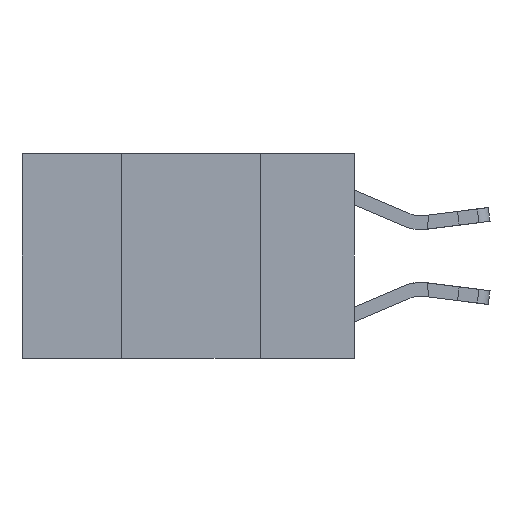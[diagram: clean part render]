
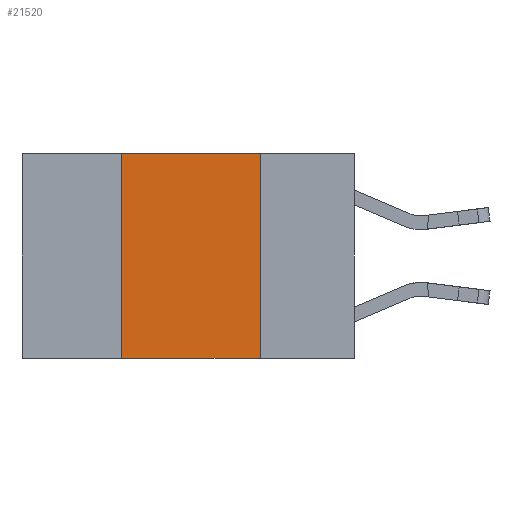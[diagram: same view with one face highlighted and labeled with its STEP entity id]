
A CAD part, left-side view. The second image highlights one B-rep face of the part: STEP entity #21520.
In plain terms, the highlighted planar face has unit normal (-1, 0, 0).
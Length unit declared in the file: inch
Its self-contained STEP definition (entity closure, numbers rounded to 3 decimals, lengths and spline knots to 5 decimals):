
#1584 = DIRECTION ( 'NONE',  ( 0., 0., 1. ) ) ;
#1764 = CARTESIAN_POINT ( 'NONE',  ( 0., 0.6, 0. ) ) ;
#3880 = AXIS2_PLACEMENT_3D ( 'NONE', #1764, #25860, #23406 ) ;
#3926 = PLANE ( 'NONE',  #3880 ) ;
#3977 = VERTEX_POINT ( 'NONE', #17524 ) ;
#4005 = LINE ( 'NONE', #19149, #17135 ) ;
#4527 = VERTEX_POINT ( 'NONE', #25700 ) ;
#5379 = CARTESIAN_POINT ( 'NONE',  ( 0., 0.6, 0. ) ) ;
#5884 = LINE ( 'NONE', #21220, #24998 ) ;
#6256 = ORIENTED_EDGE ( 'NONE', *, *, #8584, .F. ) ;
#6330 = EDGE_LOOP ( 'NONE', ( #6256, #14389, #12923, #17954 ) ) ;
#7121 = DIRECTION ( 'NONE',  ( 0., 0., -1. ) ) ;
#7507 = DIRECTION ( 'NONE',  ( 0., -1., 0. ) ) ;
#8006 = EDGE_CURVE ( 'NONE', #17772, #4527, #5884, .T. ) ;
#8355 = CARTESIAN_POINT ( 'NONE',  ( 0., 0.17, -0.37 ) ) ;
#8414 = EDGE_CURVE ( 'NONE', #17772, #23337, #4005, .T. ) ;
#8584 = EDGE_CURVE ( 'NONE', #3977, #23337, #15847, .T. ) ;
#10633 = FACE_OUTER_BOUND ( 'NONE', #6330, .T. ) ;
#12923 = ORIENTED_EDGE ( 'NONE', *, *, #8006, .F. ) ;
#13916 = CARTESIAN_POINT ( 'NONE',  ( 0., 0.42, -0.37 ) ) ;
#14389 = ORIENTED_EDGE ( 'NONE', *, *, #17195, .F. ) ;
#15847 = LINE ( 'NONE', #17856, #17683 ) ;
#16482 = VECTOR ( 'NONE', #7507, 39.37008 ) ;
#17135 = VECTOR ( 'NONE', #23484, 39.37008 ) ;
#17195 = EDGE_CURVE ( 'NONE', #4527, #3977, #27039, .T. ) ;
#17524 = CARTESIAN_POINT ( 'NONE',  ( 0., 0.17, 0. ) ) ;
#17683 = VECTOR ( 'NONE', #7121, 39.37008 ) ;
#17772 = VERTEX_POINT ( 'NONE', #13916 ) ;
#17856 = CARTESIAN_POINT ( 'NONE',  ( 0., 0.17, 0. ) ) ;
#17954 = ORIENTED_EDGE ( 'NONE', *, *, #8414, .T. ) ;
#19149 = CARTESIAN_POINT ( 'NONE',  ( 0., 0.6, -0.37 ) ) ;
#21220 = CARTESIAN_POINT ( 'NONE',  ( 0., 0.42, 0. ) ) ;
#21520 = ADVANCED_FACE ( 'NONE', ( #10633 ), #3926, .F. ) ;
#23337 = VERTEX_POINT ( 'NONE', #8355 ) ;
#23406 = DIRECTION ( 'NONE',  ( 0., 0., -1. ) ) ;
#23484 = DIRECTION ( 'NONE',  ( 0., -1., 0. ) ) ;
#24998 = VECTOR ( 'NONE', #1584, 39.37008 ) ;
#25700 = CARTESIAN_POINT ( 'NONE',  ( 0., 0.42, 0. ) ) ;
#25860 = DIRECTION ( 'NONE',  ( 1., 0., 0. ) ) ;
#27039 = LINE ( 'NONE', #5379, #16482 ) ;
